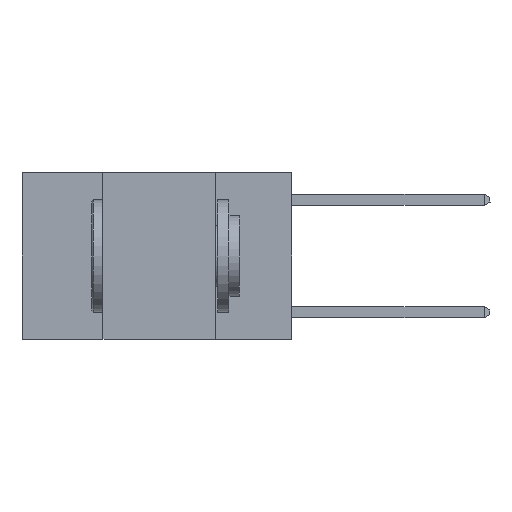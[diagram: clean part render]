
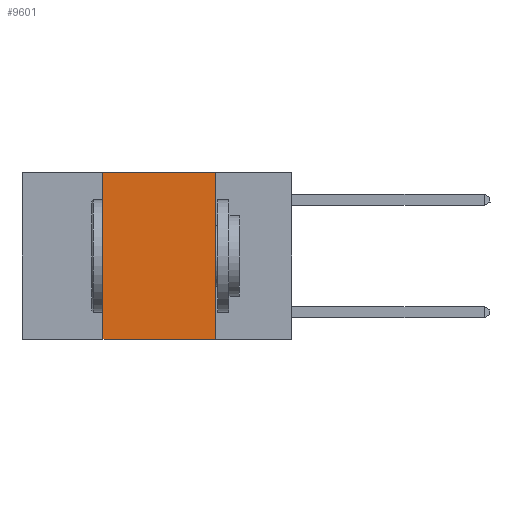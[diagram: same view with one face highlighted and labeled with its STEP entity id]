
A CAD part, left-side view. The second image highlights one B-rep face of the part: STEP entity #9601.
In plain terms, the highlighted planar face has unit normal (-1, 0, 0).
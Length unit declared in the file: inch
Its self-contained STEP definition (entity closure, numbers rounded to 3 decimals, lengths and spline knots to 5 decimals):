
#52 = DIRECTION ( 'NONE',  ( 0., -1., 0. ) ) ;
#144 = CARTESIAN_POINT ( 'NONE',  ( 0., 0.6, 0. ) ) ;
#670 = VERTEX_POINT ( 'NONE', #6612 ) ;
#860 = DIRECTION ( 'NONE',  ( 0., 0., -1. ) ) ;
#1188 = EDGE_LOOP ( 'NONE', ( #2229, #2362, #2381, #2995 ) ) ;
#1479 = CARTESIAN_POINT ( 'NONE',  ( 0., 0.17, 0. ) ) ;
#1662 = EDGE_CURVE ( 'NONE', #5830, #670, #15023, .T. ) ;
#2229 = ORIENTED_EDGE ( 'NONE', *, *, #3370, .F. ) ;
#2362 = ORIENTED_EDGE ( 'NONE', *, *, #4333, .F. ) ;
#2381 = ORIENTED_EDGE ( 'NONE', *, *, #2928, .F. ) ;
#2928 = EDGE_CURVE ( 'NONE', #5830, #3553, #7821, .T. ) ;
#2995 = ORIENTED_EDGE ( 'NONE', *, *, #1662, .T. ) ;
#3329 = CARTESIAN_POINT ( 'NONE',  ( 0., 0.6, 0. ) ) ;
#3337 = VECTOR ( 'NONE', #52, 39.37008 ) ;
#3370 = EDGE_CURVE ( 'NONE', #8624, #670, #5842, .T. ) ;
#3553 = VERTEX_POINT ( 'NONE', #10390 ) ;
#4333 = EDGE_CURVE ( 'NONE', #3553, #8624, #9556, .T. ) ;
#4558 = DIRECTION ( 'NONE',  ( 1., 0., 0. ) ) ;
#4722 = VECTOR ( 'NONE', #7118, 39.37008 ) ;
#4749 = CARTESIAN_POINT ( 'NONE',  ( 0., 0.42, -0.37 ) ) ;
#4964 = FACE_OUTER_BOUND ( 'NONE', #1188, .T. ) ;
#5830 = VERTEX_POINT ( 'NONE', #4749 ) ;
#5842 = LINE ( 'NONE', #1479, #11936 ) ;
#6612 = CARTESIAN_POINT ( 'NONE',  ( 0., 0.17, -0.37 ) ) ;
#7118 = DIRECTION ( 'NONE',  ( 0., 0., 1. ) ) ;
#7821 = LINE ( 'NONE', #14965, #4722 ) ;
#8624 = VERTEX_POINT ( 'NONE', #13284 ) ;
#9303 = AXIS2_PLACEMENT_3D ( 'NONE', #3329, #4558, #12621 ) ;
#9556 = LINE ( 'NONE', #144, #3337 ) ;
#9601 = ADVANCED_FACE ( 'NONE', ( #4964 ), #10308, .F. ) ;
#10308 = PLANE ( 'NONE',  #9303 ) ;
#10390 = CARTESIAN_POINT ( 'NONE',  ( 0., 0.42, 0. ) ) ;
#11534 = CARTESIAN_POINT ( 'NONE',  ( 0., 0.6, -0.37 ) ) ;
#11547 = DIRECTION ( 'NONE',  ( 0., -1., 0. ) ) ;
#11936 = VECTOR ( 'NONE', #860, 39.37008 ) ;
#12074 = VECTOR ( 'NONE', #11547, 39.37008 ) ;
#12621 = DIRECTION ( 'NONE',  ( 0., 0., -1. ) ) ;
#13284 = CARTESIAN_POINT ( 'NONE',  ( 0., 0.17, 0. ) ) ;
#14965 = CARTESIAN_POINT ( 'NONE',  ( 0., 0.42, 0. ) ) ;
#15023 = LINE ( 'NONE', #11534, #12074 ) ;
